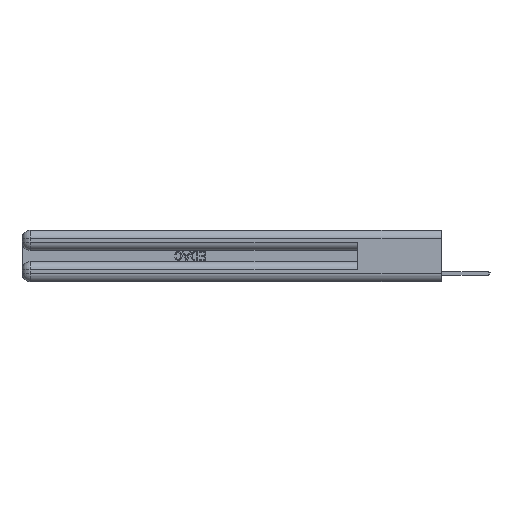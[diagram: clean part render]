
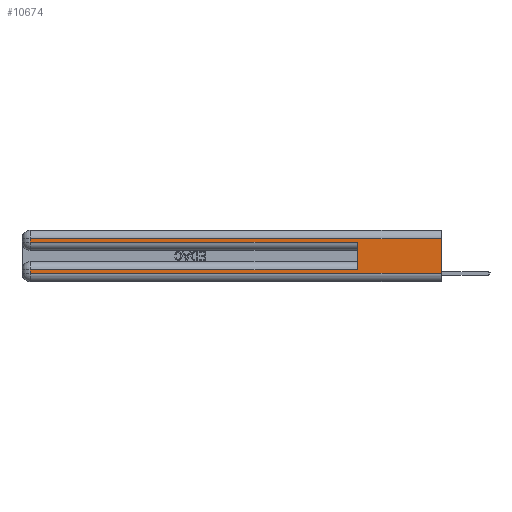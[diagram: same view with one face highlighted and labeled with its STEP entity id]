
A CAD part, left-side view. The second image highlights one B-rep face of the part: STEP entity #10674.
In plain terms, the highlighted planar face has unit normal (-1, 0, 0).
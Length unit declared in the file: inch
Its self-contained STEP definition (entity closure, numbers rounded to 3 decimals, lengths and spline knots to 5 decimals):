
#45 = VECTOR ( 'NONE', #12932, 39.37008 ) ;
#1705 = LINE ( 'NONE', #14739, #45 ) ;
#2035 = CARTESIAN_POINT ( 'NONE',  ( 0., 2.94, 0.285 ) ) ;
#2290 = CARTESIAN_POINT ( 'NONE',  ( 0., 2.94, 0.31 ) ) ;
#2480 = CARTESIAN_POINT ( 'NONE',  ( 0., 2.94, 0.06 ) ) ;
#2661 = VECTOR ( 'NONE', #24357, 39.37008 ) ;
#3667 = DIRECTION ( 'NONE',  ( 0., 1., 0. ) ) ;
#3800 = DIRECTION ( 'NONE',  ( 0., -1., 0. ) ) ;
#4257 = VECTOR ( 'NONE', #23236, 39.37008 ) ;
#4501 = LINE ( 'NONE', #11257, #2661 ) ;
#4584 = ORIENTED_EDGE ( 'NONE', *, *, #29031, .T. ) ;
#5162 = LINE ( 'NONE', #14149, #4257 ) ;
#5998 = CARTESIAN_POINT ( 'NONE',  ( 0., 0., 0.06 ) ) ;
#6343 = EDGE_CURVE ( 'NONE', #11081, #24881, #12250, .T. ) ;
#7939 = ORIENTED_EDGE ( 'NONE', *, *, #11713, .T. ) ;
#8255 = VECTOR ( 'NONE', #3667, 39.37008 ) ;
#8303 = CARTESIAN_POINT ( 'NONE',  ( 0., 2.94, 0.085 ) ) ;
#8453 = DIRECTION ( 'NONE',  ( 0., 0., -1. ) ) ;
#8664 = EDGE_LOOP ( 'NONE', ( #21389, #7939, #25897, #4584, #27074, #23839, #20415, #28495 ) ) ;
#9308 = VERTEX_POINT ( 'NONE', #20901 ) ;
#9646 = VECTOR ( 'NONE', #3800, 39.37008 ) ;
#10674 = ADVANCED_FACE ( 'NONE', ( #21663 ), #19265, .F. ) ;
#10896 = CARTESIAN_POINT ( 'NONE',  ( 0., 0.6, 0.085 ) ) ;
#11081 = VERTEX_POINT ( 'NONE', #10896 ) ;
#11257 = CARTESIAN_POINT ( 'NONE',  ( 0., 0., 0.37 ) ) ;
#11713 = EDGE_CURVE ( 'NONE', #9308, #17862, #23831, .T. ) ;
#12145 = DIRECTION ( 'NONE',  ( 0., 0., -1. ) ) ;
#12207 = VERTEX_POINT ( 'NONE', #5998 ) ;
#12250 = LINE ( 'NONE', #21377, #12591 ) ;
#12309 = EDGE_CURVE ( 'NONE', #9308, #12207, #4501, .T. ) ;
#12519 = VERTEX_POINT ( 'NONE', #2480 ) ;
#12591 = VECTOR ( 'NONE', #24744, 39.37008 ) ;
#12838 = CARTESIAN_POINT ( 'NONE',  ( 0., 0., 0.37 ) ) ;
#12932 = DIRECTION ( 'NONE',  ( 0., -1., 0. ) ) ;
#13317 = VERTEX_POINT ( 'NONE', #8303 ) ;
#14006 = EDGE_CURVE ( 'NONE', #11081, #13317, #19234, .T. ) ;
#14149 = CARTESIAN_POINT ( 'NONE',  ( 0., 2.94, 0.37 ) ) ;
#14739 = CARTESIAN_POINT ( 'NONE',  ( 0., 0., 0.06 ) ) ;
#14808 = VECTOR ( 'NONE', #12145, 39.37008 ) ;
#14911 = CARTESIAN_POINT ( 'NONE',  ( 0., 0., 0.31 ) ) ;
#15888 = EDGE_CURVE ( 'NONE', #17862, #20814, #5162, .T. ) ;
#16859 = DIRECTION ( 'NONE',  ( 0., 1., 0. ) ) ;
#17862 = VERTEX_POINT ( 'NONE', #2290 ) ;
#18870 = VECTOR ( 'NONE', #16859, 39.37008 ) ;
#19063 = EDGE_CURVE ( 'NONE', #12519, #12207, #1705, .T. ) ;
#19234 = LINE ( 'NONE', #28225, #18870 ) ;
#19265 = PLANE ( 'NONE',  #26617 ) ;
#20415 = ORIENTED_EDGE ( 'NONE', *, *, #26924, .T. ) ;
#20814 = VERTEX_POINT ( 'NONE', #2035 ) ;
#20901 = CARTESIAN_POINT ( 'NONE',  ( 0., 0., 0.31 ) ) ;
#21377 = CARTESIAN_POINT ( 'NONE',  ( 0., 0.6, 0.145 ) ) ;
#21384 = CARTESIAN_POINT ( 'NONE',  ( 0., 0.6, 0.285 ) ) ;
#21389 = ORIENTED_EDGE ( 'NONE', *, *, #12309, .F. ) ;
#21663 = FACE_OUTER_BOUND ( 'NONE', #8664, .T. ) ;
#21742 = LINE ( 'NONE', #24250, #9646 ) ;
#23236 = DIRECTION ( 'NONE',  ( 0., 0., -1. ) ) ;
#23450 = CARTESIAN_POINT ( 'NONE',  ( 0., 2.94, 0.37 ) ) ;
#23831 = LINE ( 'NONE', #14911, #8255 ) ;
#23839 = ORIENTED_EDGE ( 'NONE', *, *, #14006, .T. ) ;
#24250 = CARTESIAN_POINT ( 'NONE',  ( 0., 0., 0.285 ) ) ;
#24357 = DIRECTION ( 'NONE',  ( 0., 0., -1. ) ) ;
#24744 = DIRECTION ( 'NONE',  ( 0., 0., 1. ) ) ;
#24881 = VERTEX_POINT ( 'NONE', #21384 ) ;
#25897 = ORIENTED_EDGE ( 'NONE', *, *, #15888, .T. ) ;
#26617 = AXIS2_PLACEMENT_3D ( 'NONE', #12838, #28249, #8453 ) ;
#26924 = EDGE_CURVE ( 'NONE', #13317, #12519, #28413, .T. ) ;
#27074 = ORIENTED_EDGE ( 'NONE', *, *, #6343, .F. ) ;
#28225 = CARTESIAN_POINT ( 'NONE',  ( 0., 0., 0.085 ) ) ;
#28249 = DIRECTION ( 'NONE',  ( 1., 0., 0. ) ) ;
#28413 = LINE ( 'NONE', #23450, #14808 ) ;
#28495 = ORIENTED_EDGE ( 'NONE', *, *, #19063, .T. ) ;
#29031 = EDGE_CURVE ( 'NONE', #20814, #24881, #21742, .T. ) ;
